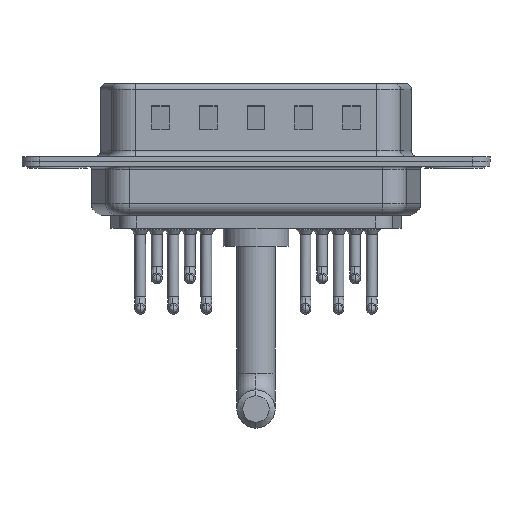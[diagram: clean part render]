
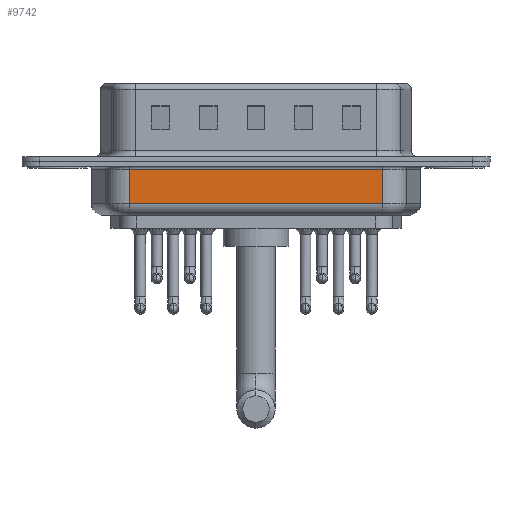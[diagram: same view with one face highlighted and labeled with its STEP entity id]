
A CAD part, front view. The second image highlights one B-rep face of the part: STEP entity #9742.
In plain terms, the highlighted planar face has unit normal (0, -1, 0).
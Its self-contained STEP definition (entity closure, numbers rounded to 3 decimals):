
#101 = PLANE ( 'NONE',  #14578 ) ;
#448 = VECTOR ( 'NONE', #19392, 1000. ) ;
#1850 = VERTEX_POINT ( 'NONE', #14098 ) ;
#3066 = VERTEX_POINT ( 'NONE', #6113 ) ;
#3892 = EDGE_CURVE ( 'NONE', #15936, #3066, #19598, .T. ) ;
#4010 = ORIENTED_EDGE ( 'NONE', *, *, #14591, .T. ) ;
#4466 = LINE ( 'NONE', #17362, #11813 ) ;
#5190 = LINE ( 'NONE', #19446, #10282 ) ;
#5259 = VERTEX_POINT ( 'NONE', #6070 ) ;
#6070 = CARTESIAN_POINT ( 'NONE',  ( 27.269, -5.35, -0.65 ) ) ;
#6113 = CARTESIAN_POINT ( 'NONE',  ( 6.031, -5.35, -0.65 ) ) ;
#6893 = ORIENTED_EDGE ( 'NONE', *, *, #9892, .T. ) ;
#6894 = CARTESIAN_POINT ( 'NONE',  ( 6.031, -5.35, -4.5 ) ) ;
#8010 = FACE_OUTER_BOUND ( 'NONE', #11940, .T. ) ;
#9509 = ORIENTED_EDGE ( 'NONE', *, *, #17208, .T. ) ;
#9742 = ADVANCED_FACE ( 'NONE', ( #8010 ), #101, .F. ) ;
#9892 = EDGE_CURVE ( 'NONE', #15936, #1850, #5190, .T. ) ;
#10052 = DIRECTION ( 'NONE',  ( 0., 0., 1. ) ) ;
#10282 = VECTOR ( 'NONE', #19156, 1000. ) ;
#10358 = LINE ( 'NONE', #15036, #19376 ) ;
#11813 = VECTOR ( 'NONE', #14120, 1000. ) ;
#11940 = EDGE_LOOP ( 'NONE', ( #17303, #6893, #4010, #9509 ) ) ;
#14098 = CARTESIAN_POINT ( 'NONE',  ( 27.269, -5.35, -3.5 ) ) ;
#14120 = DIRECTION ( 'NONE',  ( -1., 0., 0. ) ) ;
#14247 = DIRECTION ( 'NONE',  ( 0., 1., 0. ) ) ;
#14578 = AXIS2_PLACEMENT_3D ( 'NONE', #18640, #14247, #17065 ) ;
#14591 = EDGE_CURVE ( 'NONE', #1850, #5259, #10358, .T. ) ;
#15036 = CARTESIAN_POINT ( 'NONE',  ( 27.269, -5.35, -4.5 ) ) ;
#15936 = VERTEX_POINT ( 'NONE', #17237 ) ;
#17065 = DIRECTION ( 'NONE',  ( 0., 0., 1. ) ) ;
#17208 = EDGE_CURVE ( 'NONE', #5259, #3066, #4466, .T. ) ;
#17237 = CARTESIAN_POINT ( 'NONE',  ( 6.031, -5.35, -3.5 ) ) ;
#17303 = ORIENTED_EDGE ( 'NONE', *, *, #3892, .F. ) ;
#17362 = CARTESIAN_POINT ( 'NONE',  ( 6.031, -5.35, -0.65 ) ) ;
#18640 = CARTESIAN_POINT ( 'NONE',  ( 6.031, -5.35, -4.5 ) ) ;
#19156 = DIRECTION ( 'NONE',  ( 1., 0., 0. ) ) ;
#19376 = VECTOR ( 'NONE', #10052, 1000. ) ;
#19392 = DIRECTION ( 'NONE',  ( 0., 0., 1. ) ) ;
#19446 = CARTESIAN_POINT ( 'NONE',  ( 6.031, -5.35, -3.5 ) ) ;
#19598 = LINE ( 'NONE', #6894, #448 ) ;
